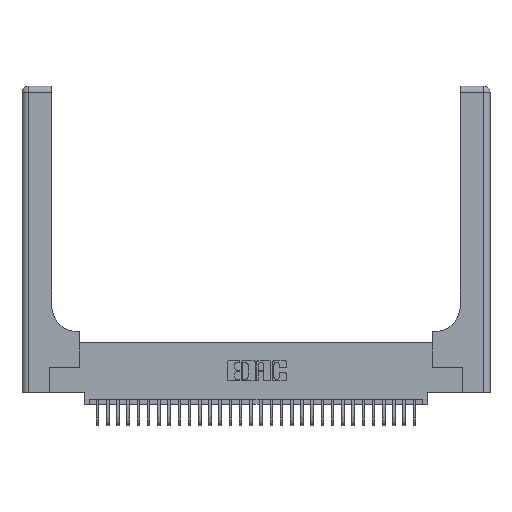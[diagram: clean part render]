
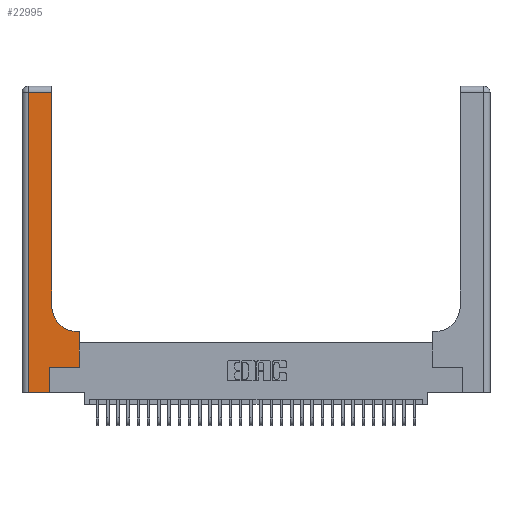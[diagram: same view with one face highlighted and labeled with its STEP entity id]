
A CAD part, top view. The second image highlights one B-rep face of the part: STEP entity #22995.
In plain terms, the highlighted planar face has unit normal (0, 0, 1).
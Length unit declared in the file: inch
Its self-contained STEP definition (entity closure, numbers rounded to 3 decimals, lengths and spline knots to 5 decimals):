
#1058 = ORIENTED_EDGE ( 'NONE', *, *, #11707, .T. ) ;
#1221 = VERTEX_POINT ( 'NONE', #19575 ) ;
#1679 = LINE ( 'NONE', #26368, #20670 ) ;
#1695 = CARTESIAN_POINT ( 'NONE',  ( 0.06, 3., 0.37 ) ) ;
#2504 = ORIENTED_EDGE ( 'NONE', *, *, #16732, .T. ) ;
#2596 = VECTOR ( 'NONE', #27781, 39.37008 ) ;
#2626 = DIRECTION ( 'NONE',  ( 1., 0., 0. ) ) ;
#2653 = DIRECTION ( 'NONE',  ( 1., 0., 0. ) ) ;
#2708 = CARTESIAN_POINT ( 'NONE',  ( 0.2915, 0.6, 0.37 ) ) ;
#2806 = EDGE_CURVE ( 'NONE', #9421, #29939, #14987, .T. ) ;
#3054 = CARTESIAN_POINT ( 'NONE',  ( 0.5415, 0.85, 0.37 ) ) ;
#3101 = ORIENTED_EDGE ( 'NONE', *, *, #26729, .T. ) ;
#3468 = DIRECTION ( 'NONE',  ( 0., 1., 0. ) ) ;
#3705 = CARTESIAN_POINT ( 'NONE',  ( 0., 0., 0.37 ) ) ;
#4304 = VERTEX_POINT ( 'NONE', #25551 ) ;
#4379 = ORIENTED_EDGE ( 'NONE', *, *, #11162, .T. ) ;
#6102 = EDGE_CURVE ( 'NONE', #4304, #20422, #29073, .T. ) ;
#6422 = VECTOR ( 'NONE', #3468, 39.37008 ) ;
#6934 = VECTOR ( 'NONE', #13907, 39.37008 ) ;
#7488 = LINE ( 'NONE', #2708, #29691 ) ;
#7642 = EDGE_CURVE ( 'NONE', #11012, #9955, #11664, .T. ) ;
#7820 = PLANE ( 'NONE',  #17370 ) ;
#8048 = DIRECTION ( 'NONE',  ( 0., 0., -1. ) ) ;
#8483 = CARTESIAN_POINT ( 'NONE',  ( 0.5585, 0.25, 0.37 ) ) ;
#8670 = VERTEX_POINT ( 'NONE', #9408 ) ;
#9408 = CARTESIAN_POINT ( 'NONE',  ( 0.5585, 0.25, 0.37 ) ) ;
#9421 = VERTEX_POINT ( 'NONE', #33151 ) ;
#9955 = VERTEX_POINT ( 'NONE', #15504 ) ;
#10488 = FACE_OUTER_BOUND ( 'NONE', #14524, .T. ) ;
#10636 = DIRECTION ( 'NONE',  ( -1., 0., 0. ) ) ;
#10718 = DIRECTION ( 'NONE',  ( -1., 0., 0. ) ) ;
#11012 = VERTEX_POINT ( 'NONE', #13348 ) ;
#11074 = LINE ( 'NONE', #1695, #2596 ) ;
#11162 = EDGE_CURVE ( 'NONE', #11933, #8670, #33244, .T. ) ;
#11313 = ORIENTED_EDGE ( 'NONE', *, *, #6102, .T. ) ;
#11664 = LINE ( 'NONE', #20977, #23799 ) ;
#11707 = EDGE_CURVE ( 'NONE', #8670, #1221, #11769, .T. ) ;
#11769 = LINE ( 'NONE', #8483, #6934 ) ;
#11933 = VERTEX_POINT ( 'NONE', #32749 ) ;
#13348 = CARTESIAN_POINT ( 'NONE',  ( 0.2915, 2.94, 0.37 ) ) ;
#13372 = CARTESIAN_POINT ( 'NONE',  ( 0.269, 0.25, 0.37 ) ) ;
#13789 = DIRECTION ( 'NONE',  ( 1., 0., 0. ) ) ;
#13907 = DIRECTION ( 'NONE',  ( 0., 1., 0. ) ) ;
#14524 = EDGE_LOOP ( 'NONE', ( #16225, #21861, #2504, #11313, #18430, #4379, #1058, #3101, #16108 ) ) ;
#14738 = DIRECTION ( 'NONE',  ( -1., 0., 0. ) ) ;
#14939 = LINE ( 'NONE', #27052, #6422 ) ;
#14987 = CIRCLE ( 'NONE', #23642, 0.25 ) ;
#15493 = DIRECTION ( 'NONE',  ( 0., 0., -1. ) ) ;
#15504 = CARTESIAN_POINT ( 'NONE',  ( 0.06, 2.94, 0.37 ) ) ;
#16108 = ORIENTED_EDGE ( 'NONE', *, *, #2806, .T. ) ;
#16225 = ORIENTED_EDGE ( 'NONE', *, *, #29844, .T. ) ;
#16596 = CARTESIAN_POINT ( 'NONE',  ( 0.2915, 0.85, 0.37 ) ) ;
#16732 = EDGE_CURVE ( 'NONE', #9955, #4304, #11074, .T. ) ;
#17370 = AXIS2_PLACEMENT_3D ( 'NONE', #23524, #8048, #10636 ) ;
#18430 = ORIENTED_EDGE ( 'NONE', *, *, #22007, .T. ) ;
#18633 = DIRECTION ( 'NONE',  ( 0., 1., 0. ) ) ;
#19575 = CARTESIAN_POINT ( 'NONE',  ( 0.5585, 0.6, 0.37 ) ) ;
#20422 = VERTEX_POINT ( 'NONE', #32904 ) ;
#20670 = VECTOR ( 'NONE', #18633, 39.37008 ) ;
#20977 = CARTESIAN_POINT ( 'NONE',  ( 0., 2.94, 0.37 ) ) ;
#21861 = ORIENTED_EDGE ( 'NONE', *, *, #7642, .T. ) ;
#22007 = EDGE_CURVE ( 'NONE', #20422, #11933, #1679, .T. ) ;
#22995 = ADVANCED_FACE ( 'NONE', ( #10488 ), #7820, .F. ) ;
#23524 = CARTESIAN_POINT ( 'NONE',  ( 0., 3., 0.37 ) ) ;
#23642 = AXIS2_PLACEMENT_3D ( 'NONE', #3054, #15493, #2626 ) ;
#23799 = VECTOR ( 'NONE', #14738, 39.37008 ) ;
#25551 = CARTESIAN_POINT ( 'NONE',  ( 0.06, 0., 0.37 ) ) ;
#26368 = CARTESIAN_POINT ( 'NONE',  ( 0.269, 0., 0.37 ) ) ;
#26374 = VECTOR ( 'NONE', #2653, 39.37008 ) ;
#26729 = EDGE_CURVE ( 'NONE', #1221, #9421, #7488, .T. ) ;
#27052 = CARTESIAN_POINT ( 'NONE',  ( 0.2915, 3., 0.37 ) ) ;
#27781 = DIRECTION ( 'NONE',  ( 0., -1., 0. ) ) ;
#29073 = LINE ( 'NONE', #3705, #31476 ) ;
#29691 = VECTOR ( 'NONE', #10718, 39.37008 ) ;
#29844 = EDGE_CURVE ( 'NONE', #29939, #11012, #14939, .T. ) ;
#29939 = VERTEX_POINT ( 'NONE', #16596 ) ;
#31476 = VECTOR ( 'NONE', #13789, 39.37008 ) ;
#32749 = CARTESIAN_POINT ( 'NONE',  ( 0.269, 0.25, 0.37 ) ) ;
#32904 = CARTESIAN_POINT ( 'NONE',  ( 0.269, 0., 0.37 ) ) ;
#33151 = CARTESIAN_POINT ( 'NONE',  ( 0.5415, 0.6, 0.37 ) ) ;
#33244 = LINE ( 'NONE', #13372, #26374 ) ;
